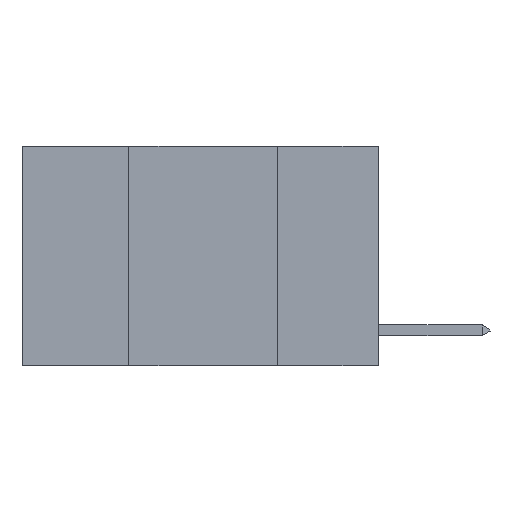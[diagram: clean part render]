
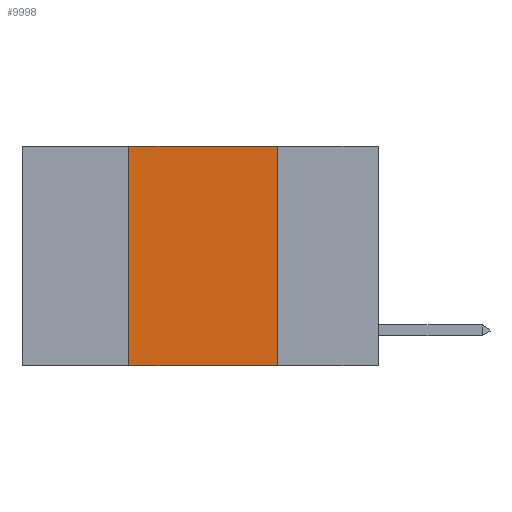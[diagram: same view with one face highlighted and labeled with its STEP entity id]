
A CAD part, left-side view. The second image highlights one B-rep face of the part: STEP entity #9998.
In plain terms, the highlighted planar face has unit normal (-1, 0, 0).
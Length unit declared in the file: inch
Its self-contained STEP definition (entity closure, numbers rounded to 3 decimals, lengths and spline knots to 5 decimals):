
#1042 = VERTEX_POINT ( 'NONE', #12746 ) ;
#1772 = LINE ( 'NONE', #2049, #2107 ) ;
#2049 = CARTESIAN_POINT ( 'NONE',  ( 0., 0.6, 0. ) ) ;
#2107 = VECTOR ( 'NONE', #9343, 39.37008 ) ;
#2504 = EDGE_LOOP ( 'NONE', ( #11192, #8476, #5549, #8285 ) ) ;
#2731 = DIRECTION ( 'NONE',  ( 0., -1., 0. ) ) ;
#2746 = CARTESIAN_POINT ( 'NONE',  ( 0., 0.17, 0. ) ) ;
#2806 = LINE ( 'NONE', #6934, #10444 ) ;
#2912 = CARTESIAN_POINT ( 'NONE',  ( 0., 0.17, 0. ) ) ;
#4210 = CARTESIAN_POINT ( 'NONE',  ( 0., 0.42, 0. ) ) ;
#4357 = LINE ( 'NONE', #5881, #7110 ) ;
#5086 = PLANE ( 'NONE',  #9181 ) ;
#5323 = VERTEX_POINT ( 'NONE', #2746 ) ;
#5549 = ORIENTED_EDGE ( 'NONE', *, *, #9281, .F. ) ;
#5881 = CARTESIAN_POINT ( 'NONE',  ( 0., 0.6, -0.37 ) ) ;
#5910 = DIRECTION ( 'NONE',  ( 0., 0., 1. ) ) ;
#6034 = DIRECTION ( 'NONE',  ( 0., 0., -1. ) ) ;
#6108 = CARTESIAN_POINT ( 'NONE',  ( 0., 0.6, 0. ) ) ;
#6734 = VECTOR ( 'NONE', #6034, 39.37008 ) ;
#6934 = CARTESIAN_POINT ( 'NONE',  ( 0., 0.42, 0. ) ) ;
#7058 = LINE ( 'NONE', #2912, #6734 ) ;
#7110 = VECTOR ( 'NONE', #2731, 39.37008 ) ;
#7150 = DIRECTION ( 'NONE',  ( 0., 0., -1. ) ) ;
#7697 = FACE_OUTER_BOUND ( 'NONE', #2504, .T. ) ;
#7778 = EDGE_CURVE ( 'NONE', #1042, #7849, #4357, .T. ) ;
#7849 = VERTEX_POINT ( 'NONE', #8092 ) ;
#8092 = CARTESIAN_POINT ( 'NONE',  ( 0., 0.17, -0.37 ) ) ;
#8285 = ORIENTED_EDGE ( 'NONE', *, *, #7778, .T. ) ;
#8476 = ORIENTED_EDGE ( 'NONE', *, *, #10091, .F. ) ;
#9181 = AXIS2_PLACEMENT_3D ( 'NONE', #6108, #13290, #7150 ) ;
#9281 = EDGE_CURVE ( 'NONE', #1042, #10117, #2806, .T. ) ;
#9343 = DIRECTION ( 'NONE',  ( 0., -1., 0. ) ) ;
#9381 = EDGE_CURVE ( 'NONE', #5323, #7849, #7058, .T. ) ;
#9998 = ADVANCED_FACE ( 'NONE', ( #7697 ), #5086, .F. ) ;
#10091 = EDGE_CURVE ( 'NONE', #10117, #5323, #1772, .T. ) ;
#10117 = VERTEX_POINT ( 'NONE', #4210 ) ;
#10444 = VECTOR ( 'NONE', #5910, 39.37008 ) ;
#11192 = ORIENTED_EDGE ( 'NONE', *, *, #9381, .F. ) ;
#12746 = CARTESIAN_POINT ( 'NONE',  ( 0., 0.42, -0.37 ) ) ;
#13290 = DIRECTION ( 'NONE',  ( 1., 0., 0. ) ) ;
